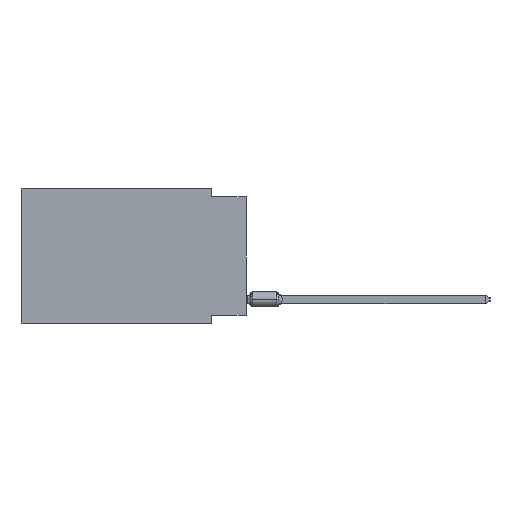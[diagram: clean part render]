
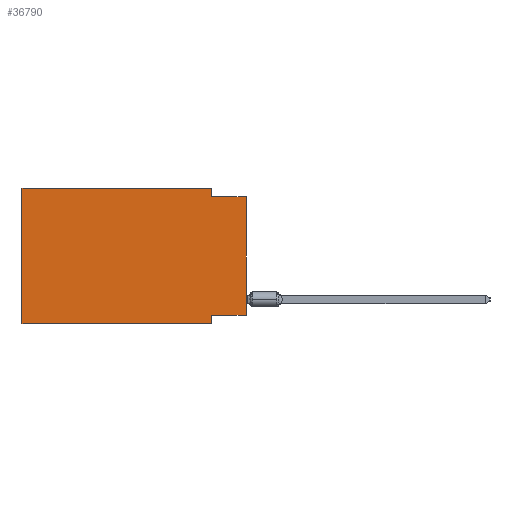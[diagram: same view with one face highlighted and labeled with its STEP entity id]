
A CAD part, left-side view. The second image highlights one B-rep face of the part: STEP entity #36790.
In plain terms, the highlighted planar face has unit normal (-1, 0, 0).
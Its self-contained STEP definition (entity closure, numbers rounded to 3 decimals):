
#522 = EDGE_CURVE ( 'NONE', #45209, #40671, #2803, .T. ) ;
#2803 = LINE ( 'NONE', #14836, #23881 ) ;
#5221 = ORIENTED_EDGE ( 'NONE', *, *, #66859, .F. ) ;
#5450 = EDGE_LOOP ( 'NONE', ( #56410, #67358, #29758, #35623, #40024, #32339, #5221, #26896 ) ) ;
#6769 = EDGE_CURVE ( 'NONE', #45209, #7319, #43505, .T. ) ;
#6920 = VERTEX_POINT ( 'NONE', #29155 ) ;
#6996 = CARTESIAN_POINT ( 'NONE',  ( 0., 2.54, -9.906 ) ) ;
#7229 = EDGE_CURVE ( 'NONE', #40671, #44270, #39603, .T. ) ;
#7319 = VERTEX_POINT ( 'NONE', #33589 ) ;
#8383 = EDGE_CURVE ( 'NONE', #44270, #22068, #60372, .T. ) ;
#8420 = CARTESIAN_POINT ( 'NONE',  ( 0., 2.54, -9.271 ) ) ;
#8689 = LINE ( 'NONE', #9054, #60120 ) ;
#9054 = CARTESIAN_POINT ( 'NONE',  ( 0., 0., 0. ) ) ;
#10245 = VECTOR ( 'NONE', #43875, 1000. ) ;
#11141 = EDGE_CURVE ( 'NONE', #6920, #74057, #32310, .T. ) ;
#14836 = CARTESIAN_POINT ( 'NONE',  ( 0., 16.383, 0. ) ) ;
#14995 = CARTESIAN_POINT ( 'NONE',  ( 0., 0., -9.271 ) ) ;
#18304 = LINE ( 'NONE', #6996, #70932 ) ;
#19027 = EDGE_CURVE ( 'NONE', #6920, #60863, #8689, .T. ) ;
#20828 = EDGE_CURVE ( 'NONE', #22068, #60863, #35234, .T. ) ;
#21077 = CARTESIAN_POINT ( 'NONE',  ( 0., 16.383, 0. ) ) ;
#22068 = VERTEX_POINT ( 'NONE', #41262 ) ;
#22930 = CARTESIAN_POINT ( 'NONE',  ( 0., 2.54, 0. ) ) ;
#23881 = VECTOR ( 'NONE', #47987, 1000. ) ;
#25913 = DIRECTION ( 'NONE',  ( 0., 0., -1. ) ) ;
#26896 = ORIENTED_EDGE ( 'NONE', *, *, #11141, .F. ) ;
#27041 = DIRECTION ( 'NONE',  ( 0., 1., 0. ) ) ;
#27957 = DIRECTION ( 'NONE',  ( 0., -1., 0. ) ) ;
#29155 = CARTESIAN_POINT ( 'NONE',  ( 0., 0., -9.271 ) ) ;
#29758 = ORIENTED_EDGE ( 'NONE', *, *, #8383, .F. ) ;
#31184 = DIRECTION ( 'NONE',  ( 1., 0., 0. ) ) ;
#32310 = LINE ( 'NONE', #14995, #45439 ) ;
#32339 = ORIENTED_EDGE ( 'NONE', *, *, #6769, .T. ) ;
#32676 = VECTOR ( 'NONE', #62354, 1000. ) ;
#33589 = CARTESIAN_POINT ( 'NONE',  ( 0., 2.54, -9.906 ) ) ;
#35234 = LINE ( 'NONE', #73994, #32676 ) ;
#35623 = ORIENTED_EDGE ( 'NONE', *, *, #7229, .F. ) ;
#35717 = FACE_OUTER_BOUND ( 'NONE', #5450, .T. ) ;
#36790 = ADVANCED_FACE ( 'NONE', ( #35717 ), #58683, .F. ) ;
#36908 = DIRECTION ( 'NONE',  ( 0., 0., 1. ) ) ;
#39603 = LINE ( 'NONE', #73082, #66612 ) ;
#40024 = ORIENTED_EDGE ( 'NONE', *, *, #522, .F. ) ;
#40671 = VERTEX_POINT ( 'NONE', #21077 ) ;
#41192 = CARTESIAN_POINT ( 'NONE',  ( 0., 16.383, -9.906 ) ) ;
#41262 = CARTESIAN_POINT ( 'NONE',  ( 0., 2.54, -0.635 ) ) ;
#43505 = LINE ( 'NONE', #44232, #10245 ) ;
#43796 = CARTESIAN_POINT ( 'NONE',  ( 0., 2.54, 0. ) ) ;
#43875 = DIRECTION ( 'NONE',  ( 0., -1., 0. ) ) ;
#44232 = CARTESIAN_POINT ( 'NONE',  ( 0., 16.383, -9.906 ) ) ;
#44270 = VERTEX_POINT ( 'NONE', #22930 ) ;
#45209 = VERTEX_POINT ( 'NONE', #41192 ) ;
#45439 = VECTOR ( 'NONE', #27041, 1000. ) ;
#47987 = DIRECTION ( 'NONE',  ( 0., 0., 1. ) ) ;
#49660 = AXIS2_PLACEMENT_3D ( 'NONE', #59070, #31184, #25913 ) ;
#56410 = ORIENTED_EDGE ( 'NONE', *, *, #19027, .T. ) ;
#58683 = PLANE ( 'NONE',  #49660 ) ;
#59070 = CARTESIAN_POINT ( 'NONE',  ( 0., 16.383, 0. ) ) ;
#60120 = VECTOR ( 'NONE', #36908, 1000. ) ;
#60372 = LINE ( 'NONE', #43796, #66767 ) ;
#60863 = VERTEX_POINT ( 'NONE', #69800 ) ;
#62354 = DIRECTION ( 'NONE',  ( 0., -1., 0. ) ) ;
#63110 = DIRECTION ( 'NONE',  ( 0., 0., -1. ) ) ;
#66612 = VECTOR ( 'NONE', #27957, 1000. ) ;
#66740 = DIRECTION ( 'NONE',  ( 0., 0., -1. ) ) ;
#66767 = VECTOR ( 'NONE', #66740, 1000. ) ;
#66859 = EDGE_CURVE ( 'NONE', #74057, #7319, #18304, .T. ) ;
#67358 = ORIENTED_EDGE ( 'NONE', *, *, #20828, .F. ) ;
#69800 = CARTESIAN_POINT ( 'NONE',  ( 0., 0., -0.635 ) ) ;
#70932 = VECTOR ( 'NONE', #63110, 1000. ) ;
#73082 = CARTESIAN_POINT ( 'NONE',  ( 0., 16.383, 0. ) ) ;
#73994 = CARTESIAN_POINT ( 'NONE',  ( 0., 0., -0.635 ) ) ;
#74057 = VERTEX_POINT ( 'NONE', #8420 ) ;
